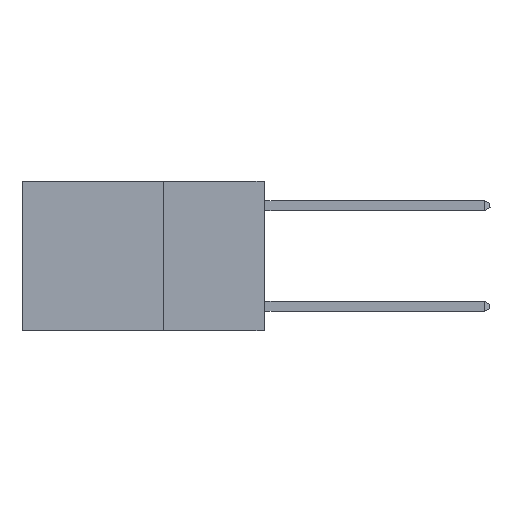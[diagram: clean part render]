
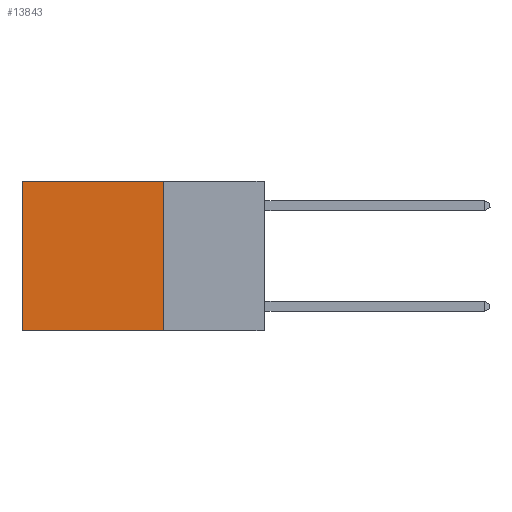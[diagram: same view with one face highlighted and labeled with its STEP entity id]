
A CAD part, left-side view. The second image highlights one B-rep face of the part: STEP entity #13843.
In plain terms, the highlighted planar face has unit normal (-1, 0, 0).
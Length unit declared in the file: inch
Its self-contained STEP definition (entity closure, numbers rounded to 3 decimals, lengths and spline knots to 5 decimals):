
#747 = EDGE_CURVE ( 'NONE', #15812, #13925, #13423, .T. ) ;
#931 = LINE ( 'NONE', #16425, #13686 ) ;
#1254 = EDGE_LOOP ( 'NONE', ( #10943, #2307, #15261, #10120 ) ) ;
#2307 = ORIENTED_EDGE ( 'NONE', *, *, #747, .F. ) ;
#2537 = CARTESIAN_POINT ( 'NONE',  ( 0.2625, 0.25, 0. ) ) ;
#2647 = CARTESIAN_POINT ( 'NONE',  ( 0.2625, 0.6, -0.37 ) ) ;
#3358 = DIRECTION ( 'NONE',  ( 0., 1., 0. ) ) ;
#3618 = DIRECTION ( 'NONE',  ( 0., 0., -1. ) ) ;
#3671 = DIRECTION ( 'NONE',  ( 0., 0., -1. ) ) ;
#4059 = VECTOR ( 'NONE', #6999, 39.37008 ) ;
#5056 = DIRECTION ( 'NONE',  ( 0., 0., -1. ) ) ;
#5433 = LINE ( 'NONE', #11212, #8814 ) ;
#5476 = AXIS2_PLACEMENT_3D ( 'NONE', #2537, #12683, #5056 ) ;
#6999 = DIRECTION ( 'NONE',  ( 0., 1., 0. ) ) ;
#7074 = CARTESIAN_POINT ( 'NONE',  ( 0.2625, 0.25, 0. ) ) ;
#7408 = EDGE_CURVE ( 'NONE', #15214, #15812, #5433, .T. ) ;
#8202 = FACE_OUTER_BOUND ( 'NONE', #1254, .T. ) ;
#8474 = VECTOR ( 'NONE', #3358, 39.37008 ) ;
#8814 = VECTOR ( 'NONE', #3618, 39.37008 ) ;
#10120 = ORIENTED_EDGE ( 'NONE', *, *, #11245, .T. ) ;
#10325 = CARTESIAN_POINT ( 'NONE',  ( 0.2625, 0.25, 0. ) ) ;
#10775 = CARTESIAN_POINT ( 'NONE',  ( 0.2625, 0.6, 0. ) ) ;
#10943 = ORIENTED_EDGE ( 'NONE', *, *, #12425, .T. ) ;
#11212 = CARTESIAN_POINT ( 'NONE',  ( 0.2625, 0.25, 0. ) ) ;
#11245 = EDGE_CURVE ( 'NONE', #15214, #12863, #11861, .T. ) ;
#11381 = PLANE ( 'NONE',  #5476 ) ;
#11861 = LINE ( 'NONE', #7074, #8474 ) ;
#12425 = EDGE_CURVE ( 'NONE', #12863, #13925, #931, .T. ) ;
#12683 = DIRECTION ( 'NONE',  ( 1., 0., 0. ) ) ;
#12741 = CARTESIAN_POINT ( 'NONE',  ( 0.2625, 0.25, -0.37 ) ) ;
#12863 = VERTEX_POINT ( 'NONE', #10775 ) ;
#13423 = LINE ( 'NONE', #13668, #4059 ) ;
#13668 = CARTESIAN_POINT ( 'NONE',  ( 0.2625, 0.25, -0.37 ) ) ;
#13686 = VECTOR ( 'NONE', #3671, 39.37008 ) ;
#13843 = ADVANCED_FACE ( 'NONE', ( #8202 ), #11381, .F. ) ;
#13925 = VERTEX_POINT ( 'NONE', #2647 ) ;
#15214 = VERTEX_POINT ( 'NONE', #10325 ) ;
#15261 = ORIENTED_EDGE ( 'NONE', *, *, #7408, .F. ) ;
#15812 = VERTEX_POINT ( 'NONE', #12741 ) ;
#16425 = CARTESIAN_POINT ( 'NONE',  ( 0.2625, 0.6, 0. ) ) ;
